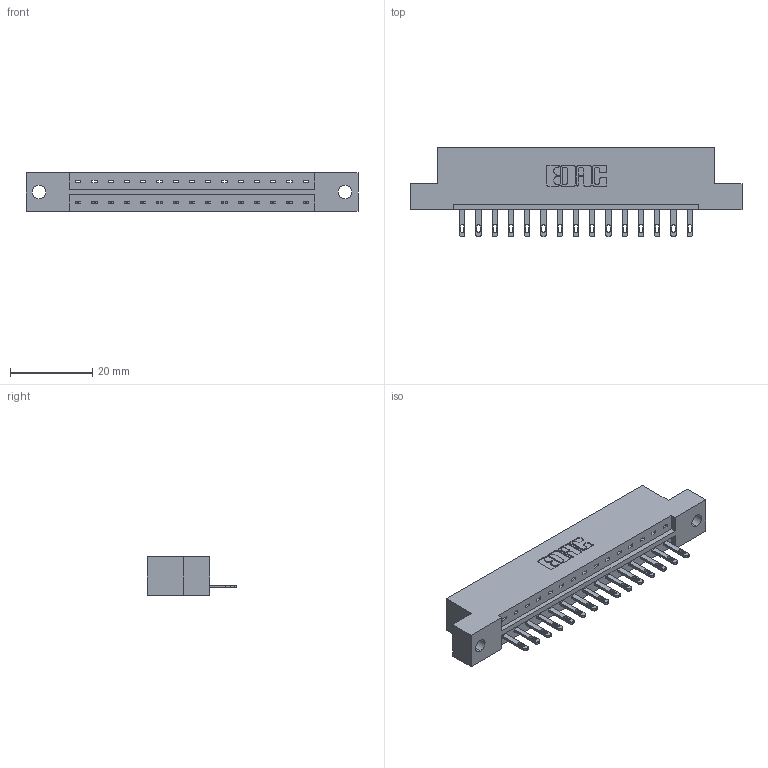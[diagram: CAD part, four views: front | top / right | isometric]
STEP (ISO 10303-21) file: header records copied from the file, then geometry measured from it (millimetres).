
FILE_DESCRIPTION (( 'STEP AP203' ), '1' );
FILE_NAME ('833-015-500-102.STEP', '2020-05-31T15:20:50', ( '' ), ( '' ), 'SwSTEP 2.0', 'SolidWorks 2020', '' );
FILE_SCHEMA (( 'CONFIG_CONTROL_DESIGN' ));
Length unit declared in the file: inch
Products named in the file (3): 833-015-500-102; 833 Part_Flush - .128 Dia; 345-292-001_345-293-100
Assembly tree (16 placements, depth 2):
  833-015-500-102
    833 Part_Flush - .128 Dia
    345-292-001_345-293-100  x15
Bounding box: 80.98 x 21.85 x 9.4 mm (x, y, z)
Volume: 7888.8 mm3; surface area: 8123 mm2
Topology: 16 solids, 16 shells, 924 faces, 2831 edges, 1886 vertices
Faces by surface type: plane 610, cylinder 314
Entity records: 12595 total; most frequent: CARTESIAN_POINT 2183, ORIENTED_EDGE 2134, DIRECTION 1897, EDGE_CURVE 1067, LINE 935, VECTOR 935, VERTEX_POINT 710, AXIS2_PLACEMENT_3D 481
